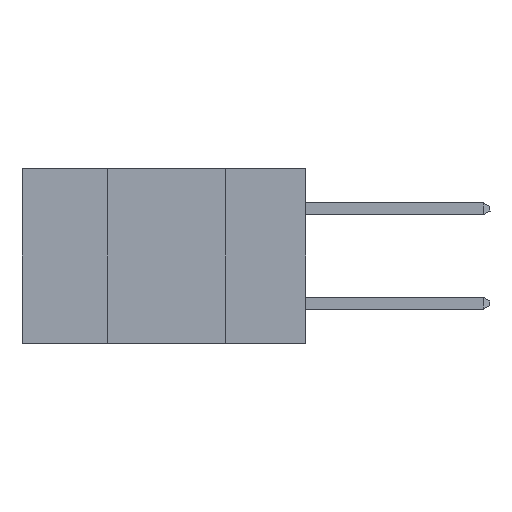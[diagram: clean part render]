
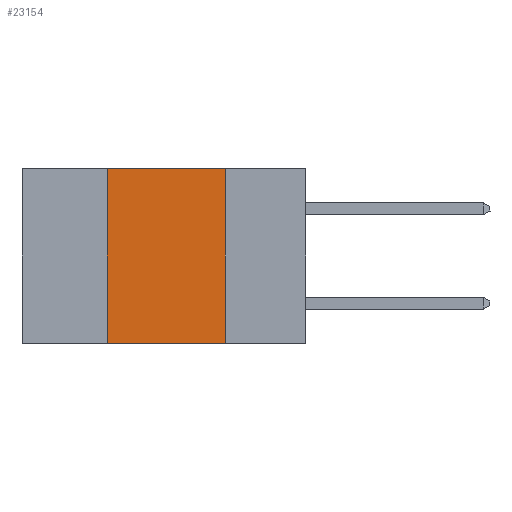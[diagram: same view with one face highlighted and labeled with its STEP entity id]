
A CAD part, left-side view. The second image highlights one B-rep face of the part: STEP entity #23154.
In plain terms, the highlighted planar face has unit normal (-1, 0, 0).
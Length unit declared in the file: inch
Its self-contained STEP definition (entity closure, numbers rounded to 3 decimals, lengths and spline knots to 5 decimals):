
#472 = LINE ( 'NONE', #1555, #20564 ) ;
#1555 = CARTESIAN_POINT ( 'NONE',  ( 0., 0.6, -0.37 ) ) ;
#2039 = CARTESIAN_POINT ( 'NONE',  ( 0., 0.17, 0. ) ) ;
#2160 = DIRECTION ( 'NONE',  ( 0., 0., -1. ) ) ;
#2302 = CARTESIAN_POINT ( 'NONE',  ( 0., 0.17, -0.37 ) ) ;
#5748 = EDGE_CURVE ( 'NONE', #23792, #20498, #30327, .T. ) ;
#8473 = FACE_OUTER_BOUND ( 'NONE', #30301, .T. ) ;
#8529 = EDGE_CURVE ( 'NONE', #11032, #23792, #31215, .T. ) ;
#8996 = AXIS2_PLACEMENT_3D ( 'NONE', #12789, #15282, #30339 ) ;
#9633 = ORIENTED_EDGE ( 'NONE', *, *, #24203, .F. ) ;
#9879 = VERTEX_POINT ( 'NONE', #2302 ) ;
#11032 = VERTEX_POINT ( 'NONE', #17436 ) ;
#12211 = VECTOR ( 'NONE', #21767, 39.37008 ) ;
#12330 = PLANE ( 'NONE',  #8996 ) ;
#12789 = CARTESIAN_POINT ( 'NONE',  ( 0., 0.6, 0. ) ) ;
#13149 = CARTESIAN_POINT ( 'NONE',  ( 0., 0.17, 0. ) ) ;
#14212 = DIRECTION ( 'NONE',  ( 0., 0., 1. ) ) ;
#14231 = DIRECTION ( 'NONE',  ( 0., -1., 0. ) ) ;
#15282 = DIRECTION ( 'NONE',  ( 1., 0., 0. ) ) ;
#17436 = CARTESIAN_POINT ( 'NONE',  ( 0., 0.42, -0.37 ) ) ;
#18631 = ORIENTED_EDGE ( 'NONE', *, *, #5748, .F. ) ;
#20498 = VERTEX_POINT ( 'NONE', #13149 ) ;
#20564 = VECTOR ( 'NONE', #14231, 39.37008 ) ;
#21279 = ORIENTED_EDGE ( 'NONE', *, *, #8529, .F. ) ;
#21767 = DIRECTION ( 'NONE',  ( 0., -1., 0. ) ) ;
#23154 = ADVANCED_FACE ( 'NONE', ( #8473 ), #12330, .F. ) ;
#23792 = VERTEX_POINT ( 'NONE', #25741 ) ;
#24019 = VECTOR ( 'NONE', #14212, 39.37008 ) ;
#24203 = EDGE_CURVE ( 'NONE', #20498, #9879, #32538, .T. ) ;
#24571 = CARTESIAN_POINT ( 'NONE',  ( 0., 0.6, 0. ) ) ;
#25741 = CARTESIAN_POINT ( 'NONE',  ( 0., 0.42, 0. ) ) ;
#26887 = VECTOR ( 'NONE', #2160, 39.37008 ) ;
#28281 = EDGE_CURVE ( 'NONE', #11032, #9879, #472, .T. ) ;
#30301 = EDGE_LOOP ( 'NONE', ( #9633, #18631, #21279, #31331 ) ) ;
#30327 = LINE ( 'NONE', #24571, #12211 ) ;
#30339 = DIRECTION ( 'NONE',  ( 0., 0., -1. ) ) ;
#31215 = LINE ( 'NONE', #32537, #24019 ) ;
#31331 = ORIENTED_EDGE ( 'NONE', *, *, #28281, .T. ) ;
#32537 = CARTESIAN_POINT ( 'NONE',  ( 0., 0.42, 0. ) ) ;
#32538 = LINE ( 'NONE', #2039, #26887 ) ;
